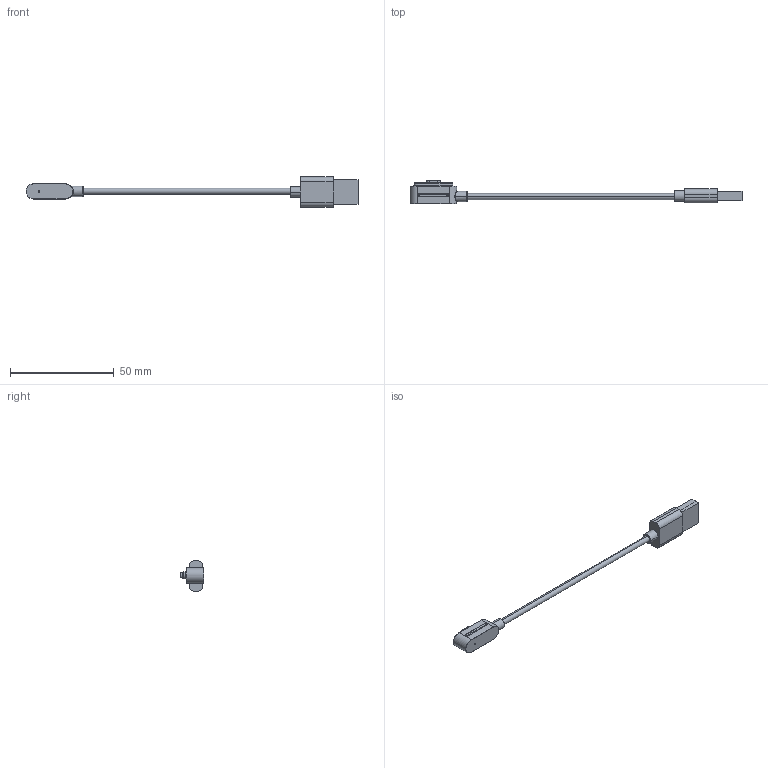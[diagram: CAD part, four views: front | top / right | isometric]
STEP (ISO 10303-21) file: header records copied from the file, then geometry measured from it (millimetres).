
FILE_DESCRIPTION (( 'STEP AP203' ), '1' );
FILE_NAME ('687G0311A100200.STEP', '2023-05-03T10:59:09', ( '' ), ( '' ), 'SwSTEP 2.0', 'SolidWorks 2020', '' );
FILE_SCHEMA (( 'CONFIG_CONTROL_DESIGN' ));
Length unit declared in the file: millimetre
Products named in the file (1): 687G0311A100200
Bounding box: 160.37 x 11.35 x 14.6 mm (x, y, z)
Volume: 4088.7 mm3; surface area: 3607.5 mm2
Topology: 6 solids, 6 shells, 214 faces, 522 edges, 335 vertices
Faces by surface type: plane 127, cylinder 53, torus 20, cone 6, sphere 6, bspline 2
Entity records: 6554 total; most frequent: CARTESIAN_POINT 1387, DIRECTION 1082, ORIENTED_EDGE 1020, EDGE_CURVE 510, AXIS2_PLACEMENT_3D 365, LINE 352, VECTOR 352, VERTEX_POINT 329
